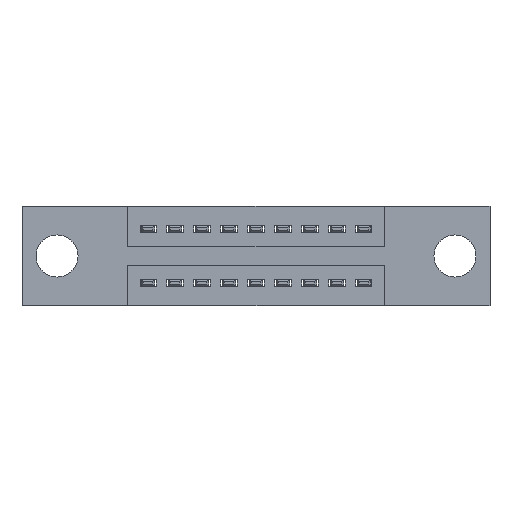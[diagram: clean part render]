
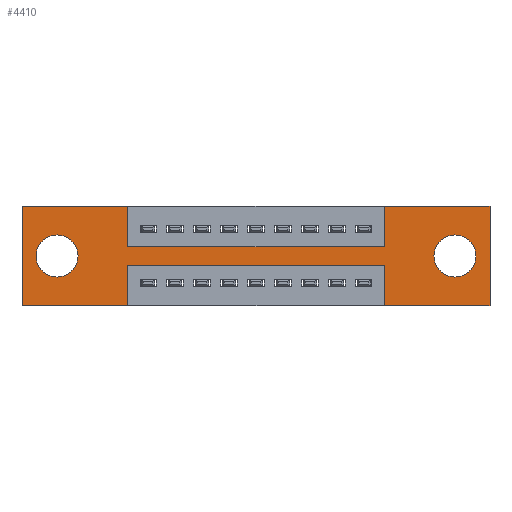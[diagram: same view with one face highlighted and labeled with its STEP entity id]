
A CAD part, front view. The second image highlights one B-rep face of the part: STEP entity #4410.
In plain terms, the highlighted planar face has unit normal (0, -1, 0).
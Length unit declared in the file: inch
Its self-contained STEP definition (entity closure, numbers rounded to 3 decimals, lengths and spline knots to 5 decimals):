
#124 = AXIS2_PLACEMENT_3D ( 'NONE', #4010, #4069, #6027 ) ;
#136 = VECTOR ( 'NONE', #10024, 39.37008 ) ;
#142 = LINE ( 'NONE', #1329, #9510 ) ;
#225 = VERTEX_POINT ( 'NONE', #1370 ) ;
#232 = EDGE_CURVE ( 'NONE', #8479, #10009, #4980, .T. ) ;
#338 = VERTEX_POINT ( 'NONE', #747 ) ;
#422 = ORIENTED_EDGE ( 'NONE', *, *, #2211, .F. ) ;
#455 = DIRECTION ( 'NONE',  ( 0., 0., 1. ) ) ;
#596 = ORIENTED_EDGE ( 'NONE', *, *, #8640, .F. ) ;
#629 = DIRECTION ( 'NONE',  ( 0., 1., 0. ) ) ;
#664 = VECTOR ( 'NONE', #9376, 39.37008 ) ;
#747 = CARTESIAN_POINT ( 'NONE',  ( 1.605, 0., -0.107 ) ) ;
#795 = VERTEX_POINT ( 'NONE', #957 ) ;
#890 = ORIENTED_EDGE ( 'NONE', *, *, #6772, .F. ) ;
#922 = EDGE_CURVE ( 'NONE', #5701, #6066, #142, .T. ) ;
#957 = CARTESIAN_POINT ( 'NONE',  ( 1.735, 0., 0. ) ) ;
#986 = EDGE_CURVE ( 'NONE', #5257, #4903, #7559, .T. ) ;
#1047 = LINE ( 'NONE', #1887, #1235 ) ;
#1110 = VECTOR ( 'NONE', #8812, 39.37008 ) ;
#1119 = ORIENTED_EDGE ( 'NONE', *, *, #986, .F. ) ;
#1159 = CARTESIAN_POINT ( 'NONE',  ( 0.3925, 0., -0.22 ) ) ;
#1162 = VERTEX_POINT ( 'NONE', #7316 ) ;
#1235 = VECTOR ( 'NONE', #3879, 39.37008 ) ;
#1329 = CARTESIAN_POINT ( 'NONE',  ( 0.3925, 0., 0. ) ) ;
#1346 = CARTESIAN_POINT ( 'NONE',  ( 1.735, 0., -0.37 ) ) ;
#1370 = CARTESIAN_POINT ( 'NONE',  ( 1.3425, 0., -0.37 ) ) ;
#1457 = VECTOR ( 'NONE', #455, 39.37008 ) ;
#1532 = VECTOR ( 'NONE', #6669, 39.37008 ) ;
#1645 = DIRECTION ( 'NONE',  ( 0., -1., 0. ) ) ;
#1688 = EDGE_CURVE ( 'NONE', #4547, #8479, #1047, .T. ) ;
#1849 = CARTESIAN_POINT ( 'NONE',  ( 0., 0., 0. ) ) ;
#1870 = CARTESIAN_POINT ( 'NONE',  ( 0.13, 0., -0.107 ) ) ;
#1887 = CARTESIAN_POINT ( 'NONE',  ( 0., 0., -0.37 ) ) ;
#1916 = CARTESIAN_POINT ( 'NONE',  ( 0., 0., -0.37 ) ) ;
#2039 = CIRCLE ( 'NONE', #9079, 0.078 ) ;
#2202 = DIRECTION ( 'NONE',  ( 1., 0., 0. ) ) ;
#2211 = EDGE_CURVE ( 'NONE', #1162, #10499, #9309, .T. ) ;
#2213 = ORIENTED_EDGE ( 'NONE', *, *, #9582, .F. ) ;
#2252 = VERTEX_POINT ( 'NONE', #1346 ) ;
#2359 = CARTESIAN_POINT ( 'NONE',  ( 0., 0., -0.37 ) ) ;
#2395 = LINE ( 'NONE', #9550, #5623 ) ;
#2423 = DIRECTION ( 'NONE',  ( 0., 0., -1. ) ) ;
#2483 = FACE_BOUND ( 'NONE', #4208, .T. ) ;
#2734 = VECTOR ( 'NONE', #3230, 39.37008 ) ;
#2890 = CARTESIAN_POINT ( 'NONE',  ( 0.3925, 0., -0.15 ) ) ;
#3036 = CARTESIAN_POINT ( 'NONE',  ( 1.3425, 0., 0. ) ) ;
#3144 = CIRCLE ( 'NONE', #8079, 0.078 ) ;
#3230 = DIRECTION ( 'NONE',  ( -1., 0., 0. ) ) ;
#3414 = LINE ( 'NONE', #9856, #8830 ) ;
#3537 = FACE_BOUND ( 'NONE', #10576, .T. ) ;
#3586 = CARTESIAN_POINT ( 'NONE',  ( 1.605, 0., -0.185 ) ) ;
#3636 = LINE ( 'NONE', #1916, #136 ) ;
#3653 = CARTESIAN_POINT ( 'NONE',  ( 0.3925, 0., -0.37 ) ) ;
#3879 = DIRECTION ( 'NONE',  ( -1., 0., 0. ) ) ;
#4010 = CARTESIAN_POINT ( 'NONE',  ( 1.605, 0., -0.185 ) ) ;
#4069 = DIRECTION ( 'NONE',  ( 0., 1., 0. ) ) ;
#4078 = VERTEX_POINT ( 'NONE', #10929 ) ;
#4195 = LINE ( 'NONE', #2890, #6153 ) ;
#4208 = EDGE_LOOP ( 'NONE', ( #9263, #6311 ) ) ;
#4246 = AXIS2_PLACEMENT_3D ( 'NONE', #2359, #1645, #2423 ) ;
#4313 = ORIENTED_EDGE ( 'NONE', *, *, #922, .F. ) ;
#4410 = ADVANCED_FACE ( 'NONE', ( #2483, #3537, #8057 ), #10577, .T. ) ;
#4519 = CARTESIAN_POINT ( 'NONE',  ( 1.735, 0., 0. ) ) ;
#4547 = VERTEX_POINT ( 'NONE', #3653 ) ;
#4605 = ORIENTED_EDGE ( 'NONE', *, *, #232, .F. ) ;
#4708 = DIRECTION ( 'NONE',  ( 0., 0., -1. ) ) ;
#4903 = VERTEX_POINT ( 'NONE', #11754 ) ;
#4915 = ORIENTED_EDGE ( 'NONE', *, *, #6124, .F. ) ;
#4952 = VERTEX_POINT ( 'NONE', #1870 ) ;
#4959 = DIRECTION ( 'NONE',  ( 0., 0., -1. ) ) ;
#4980 = LINE ( 'NONE', #6827, #1457 ) ;
#5257 = VERTEX_POINT ( 'NONE', #11443 ) ;
#5619 = CARTESIAN_POINT ( 'NONE',  ( 1.3425, 0., -0.37 ) ) ;
#5623 = VECTOR ( 'NONE', #4959, 39.37008 ) ;
#5701 = VERTEX_POINT ( 'NONE', #6946 ) ;
#5731 = LINE ( 'NONE', #5619, #664 ) ;
#5787 = EDGE_CURVE ( 'NONE', #6066, #5257, #4195, .T. ) ;
#5791 = AXIS2_PLACEMENT_3D ( 'NONE', #3586, #8301, #10146 ) ;
#5827 = DIRECTION ( 'NONE',  ( 0., 1., 0. ) ) ;
#5964 = CARTESIAN_POINT ( 'NONE',  ( 0.3925, 0., -0.15 ) ) ;
#6027 = DIRECTION ( 'NONE',  ( 0., 0., -1. ) ) ;
#6066 = VERTEX_POINT ( 'NONE', #5964 ) ;
#6124 = EDGE_CURVE ( 'NONE', #4903, #795, #3414, .T. ) ;
#6148 = ORIENTED_EDGE ( 'NONE', *, *, #11255, .F. ) ;
#6153 = VECTOR ( 'NONE', #9142, 39.37008 ) ;
#6225 = EDGE_CURVE ( 'NONE', #4078, #338, #11309, .T. ) ;
#6284 = CARTESIAN_POINT ( 'NONE',  ( 0.3925, 0., -0.22 ) ) ;
#6311 = ORIENTED_EDGE ( 'NONE', *, *, #6225, .T. ) ;
#6669 = DIRECTION ( 'NONE',  ( 0., 0., 1. ) ) ;
#6670 = CARTESIAN_POINT ( 'NONE',  ( 0., 0., 0. ) ) ;
#6772 = EDGE_CURVE ( 'NONE', #10009, #5701, #6789, .T. ) ;
#6775 = CIRCLE ( 'NONE', #124, 0.078 ) ;
#6789 = LINE ( 'NONE', #6670, #9432 ) ;
#6796 = EDGE_CURVE ( 'NONE', #4952, #7150, #3144, .T. ) ;
#6827 = CARTESIAN_POINT ( 'NONE',  ( 0., 0., 0. ) ) ;
#6946 = CARTESIAN_POINT ( 'NONE',  ( 0.3925, 0., 0. ) ) ;
#7041 = ORIENTED_EDGE ( 'NONE', *, *, #7925, .F. ) ;
#7150 = VERTEX_POINT ( 'NONE', #8435 ) ;
#7205 = LINE ( 'NONE', #4519, #1110 ) ;
#7316 = CARTESIAN_POINT ( 'NONE',  ( 1.3425, 0., -0.22 ) ) ;
#7502 = CARTESIAN_POINT ( 'NONE',  ( 0.13, 0., -0.185 ) ) ;
#7521 = EDGE_CURVE ( 'NONE', #338, #4078, #6775, .T. ) ;
#7559 = LINE ( 'NONE', #3036, #1532 ) ;
#7892 = DIRECTION ( 'NONE',  ( 0., 0., 1. ) ) ;
#7925 = EDGE_CURVE ( 'NONE', #10499, #4547, #2395, .T. ) ;
#8057 = FACE_OUTER_BOUND ( 'NONE', #10791, .T. ) ;
#8079 = AXIS2_PLACEMENT_3D ( 'NONE', #7502, #5827, #8450 ) ;
#8301 = DIRECTION ( 'NONE',  ( 0., 1., 0. ) ) ;
#8435 = CARTESIAN_POINT ( 'NONE',  ( 0.13, 0., -0.263 ) ) ;
#8450 = DIRECTION ( 'NONE',  ( 0., 0., 1. ) ) ;
#8479 = VERTEX_POINT ( 'NONE', #9929 ) ;
#8517 = ORIENTED_EDGE ( 'NONE', *, *, #1688, .F. ) ;
#8640 = EDGE_CURVE ( 'NONE', #225, #1162, #5731, .T. ) ;
#8812 = DIRECTION ( 'NONE',  ( 0., 0., -1. ) ) ;
#8830 = VECTOR ( 'NONE', #9794, 39.37008 ) ;
#9079 = AXIS2_PLACEMENT_3D ( 'NONE', #10523, #629, #7892 ) ;
#9142 = DIRECTION ( 'NONE',  ( 1., 0., 0. ) ) ;
#9263 = ORIENTED_EDGE ( 'NONE', *, *, #7521, .T. ) ;
#9309 = LINE ( 'NONE', #1159, #2734 ) ;
#9376 = DIRECTION ( 'NONE',  ( 0., 0., 1. ) ) ;
#9432 = VECTOR ( 'NONE', #2202, 39.37008 ) ;
#9510 = VECTOR ( 'NONE', #4708, 39.37008 ) ;
#9550 = CARTESIAN_POINT ( 'NONE',  ( 0.3925, 0., -0.37 ) ) ;
#9582 = EDGE_CURVE ( 'NONE', #2252, #225, #3636, .T. ) ;
#9593 = ORIENTED_EDGE ( 'NONE', *, *, #5787, .F. ) ;
#9794 = DIRECTION ( 'NONE',  ( 1., 0., 0. ) ) ;
#9856 = CARTESIAN_POINT ( 'NONE',  ( 0., 0., 0. ) ) ;
#9929 = CARTESIAN_POINT ( 'NONE',  ( 0., 0., -0.37 ) ) ;
#10009 = VERTEX_POINT ( 'NONE', #1849 ) ;
#10024 = DIRECTION ( 'NONE',  ( -1., 0., 0. ) ) ;
#10146 = DIRECTION ( 'NONE',  ( 0., 0., -1. ) ) ;
#10314 = EDGE_CURVE ( 'NONE', #7150, #4952, #2039, .T. ) ;
#10499 = VERTEX_POINT ( 'NONE', #6284 ) ;
#10523 = CARTESIAN_POINT ( 'NONE',  ( 0.13, 0., -0.185 ) ) ;
#10576 = EDGE_LOOP ( 'NONE', ( #10871, #11346 ) ) ;
#10577 = PLANE ( 'NONE',  #4246 ) ;
#10791 = EDGE_LOOP ( 'NONE', ( #7041, #422, #596, #2213, #6148, #4915, #1119, #9593, #4313, #890, #4605, #8517 ) ) ;
#10871 = ORIENTED_EDGE ( 'NONE', *, *, #6796, .T. ) ;
#10929 = CARTESIAN_POINT ( 'NONE',  ( 1.605, 0., -0.263 ) ) ;
#11255 = EDGE_CURVE ( 'NONE', #795, #2252, #7205, .T. ) ;
#11309 = CIRCLE ( 'NONE', #5791, 0.078 ) ;
#11346 = ORIENTED_EDGE ( 'NONE', *, *, #10314, .T. ) ;
#11443 = CARTESIAN_POINT ( 'NONE',  ( 1.3425, 0., -0.15 ) ) ;
#11754 = CARTESIAN_POINT ( 'NONE',  ( 1.3425, 0., 0. ) ) ;
